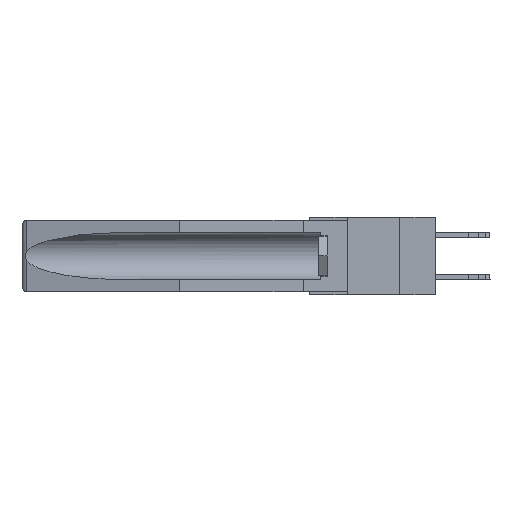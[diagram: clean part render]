
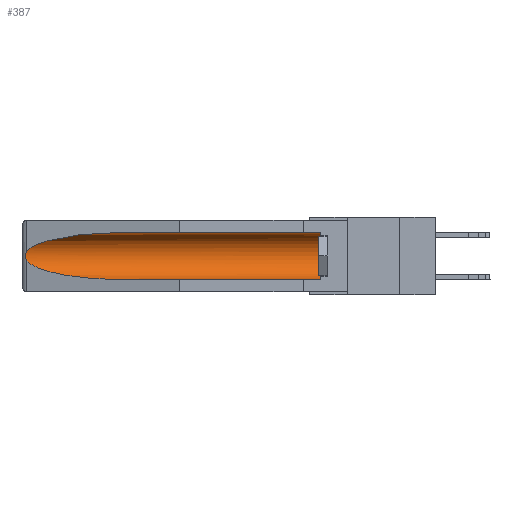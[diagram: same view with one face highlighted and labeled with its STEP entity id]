
A CAD part, left-side view. The second image highlights one B-rep face of the part: STEP entity #387.
In plain terms, the highlighted cylindrical face has radius 2.857 mm (diameter 5.715 mm), a partial arc.
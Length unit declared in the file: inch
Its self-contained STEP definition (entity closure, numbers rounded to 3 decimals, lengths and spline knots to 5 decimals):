
#278 = CARTESIAN_POINT ( 'NONE',  ( 0.155, -0.30754, -0.284 ) ) ;
#387 = ADVANCED_FACE ( 'NONE', ( #7791 ), #4352, .F. ) ;
#392 = DIRECTION ( 'NONE',  ( 0., 1., 0. ) ) ;
#547 = ORIENTED_EDGE ( 'NONE', *, *, #2767, .T. ) ;
#944 = VERTEX_POINT ( 'NONE', #14976 ) ;
#1059 = VERTEX_POINT ( 'NONE', #2539 ) ;
#2043 = CARTESIAN_POINT ( 'NONE',  ( 0.26597, 1.52961, -0.15275 ) ) ;
#2257 = VECTOR ( 'NONE', #392, 39.37008 ) ;
#2539 = CARTESIAN_POINT ( 'NONE',  ( 0.26537, 1.52718, -0.19328 ) ) ;
#2569 = EDGE_CURVE ( 'NONE', #944, #1059, #17378, .T. ) ;
#2767 = EDGE_CURVE ( 'NONE', #16362, #15933, #8404, .T. ) ;
#2847 = ORIENTED_EDGE ( 'NONE', *, *, #15312, .T. ) ;
#2925 = ORIENTED_EDGE ( 'NONE', *, *, #7594, .F. ) ;
#3388 = CARTESIAN_POINT ( 'NONE',  ( 0.2673, 1.5327, -0.16383 ) ) ;
#3452 = CARTESIAN_POINT ( 'NONE',  ( 0.2675, 1.53308, -0.17534 ) ) ;
#3769 = CARTESIAN_POINT ( 'NONE',  ( 0.21114, 1.30732, -0.059 ) ) ;
#4297 = EDGE_LOOP ( 'NONE', ( #7400, #14884, #2847, #2925, #547, #15080 ) ) ;
#4300 = EDGE_CURVE ( 'NONE', #12105, #944, #15067, .T. ) ;
#4352 = CYLINDRICAL_SURFACE ( 'NONE', #15417, 0.1125 ) ;
#4478 = DIRECTION ( 'NONE',  ( 0., 1., 0. ) ) ;
#5086 = CARTESIAN_POINT ( 'NONE',  ( 0.155, 1.07973, -0.059 ) ) ;
#5438 = CARTESIAN_POINT ( 'NONE',  ( 0.26537, 1.52718, -0.19328 ) ) ;
#7260 = DIRECTION ( 'NONE',  ( 0., 0., 1. ) ) ;
#7400 = ORIENTED_EDGE ( 'NONE', *, *, #4300, .T. ) ;
#7594 = EDGE_CURVE ( 'NONE', #16362, #12061, #15468, .T. ) ;
#7743 = CARTESIAN_POINT ( 'NONE',  ( 0.25451, 1.48313, -0.09465 ) ) ;
#7791 = FACE_OUTER_BOUND ( 'NONE', #4297, .T. ) ;
#8350 = CARTESIAN_POINT ( 'NONE',  ( 0.25451, 1.48313, -0.24835 ) ) ;
#8404 = CIRCLE ( 'NONE', #9414, 0.1125 ) ;
#9414 = AXIS2_PLACEMENT_3D ( 'NONE', #10332, #17138, #13149 ) ;
#9987 = CARTESIAN_POINT ( 'NONE',  ( 0.155, -0.30754, -0.059 ) ) ;
#10272 = CARTESIAN_POINT ( 'NONE',  ( 0.26537, 1.52718, -0.14972 ) ) ;
#10332 = CARTESIAN_POINT ( 'NONE',  ( 0.155, 0.126, -0.1715 ) ) ;
#11427 = CARTESIAN_POINT ( 'NONE',  ( 0.26537, 1.52718, -0.19328 ) ) ;
#12061 = VERTEX_POINT ( 'NONE', #16792 ) ;
#12105 = VERTEX_POINT ( 'NONE', #5086 ) ;
#12358 = CARTESIAN_POINT ( 'NONE',  ( 0.21114, 1.30732, -0.284 ) ) ;
#12684 = CARTESIAN_POINT ( 'NONE',  ( 0.155, -0.30754, -0.1715 ) ) ;
#12756 = CARTESIAN_POINT ( 'NONE',  ( 0.26655, 1.53094, -0.18657 ) ) ;
#12764 = LINE ( 'NONE', #9987, #15703 ) ;
#13149 = DIRECTION ( 'NONE',  ( 0., 0., 1. ) ) ;
#13809 = CARTESIAN_POINT ( 'NONE',  ( 0.155, 1.07973, -0.284 ) ) ;
#14308 = CARTESIAN_POINT ( 'NONE',  ( 0.2675, 1.53308, -0.16763 ) ) ;
#14505 = CARTESIAN_POINT ( 'NONE',  ( 0.155, 1.07973, -0.059 ) ) ;
#14884 = ORIENTED_EDGE ( 'NONE', *, *, #2569, .T. ) ;
#14976 = CARTESIAN_POINT ( 'NONE',  ( 0.26537, 1.52718, -0.14972 ) ) ;
#15067 =( BOUNDED_CURVE ( )  B_SPLINE_CURVE ( 3, ( #14505, #3769, #7743, #17256 ),
 .UNSPECIFIED., .F., .F. ) 
 B_SPLINE_CURVE_WITH_KNOTS ( ( 4, 4 ),
 ( 4.71239, 6.08839 ),
 .UNSPECIFIED. ) 
 CURVE ( )  GEOMETRIC_REPRESENTATION_ITEM ( )  RATIONAL_B_SPLINE_CURVE ( ( 1., 0.848, 0.848, 1. ) ) 
 REPRESENTATION_ITEM ( '' )  );
#15080 = ORIENTED_EDGE ( 'NONE', *, *, #17564, .T. ) ;
#15312 = EDGE_CURVE ( 'NONE', #1059, #12061, #16622, .T. ) ;
#15403 = CARTESIAN_POINT ( 'NONE',  ( 0.26597, 1.5296, -0.19026 ) ) ;
#15417 = AXIS2_PLACEMENT_3D ( 'NONE', #12684, #4478, #7260 ) ;
#15468 = LINE ( 'NONE', #278, #2257 ) ;
#15663 = CARTESIAN_POINT ( 'NONE',  ( 0.2673, 1.53269, -0.17917 ) ) ;
#15703 = VECTOR ( 'NONE', #16709, 39.37008 ) ;
#15933 = VERTEX_POINT ( 'NONE', #16894 ) ;
#16184 = CARTESIAN_POINT ( 'NONE',  ( 0.155, 0.126, -0.284 ) ) ;
#16362 = VERTEX_POINT ( 'NONE', #16184 ) ;
#16622 =( BOUNDED_CURVE ( )  B_SPLINE_CURVE ( 3, ( #5438, #8350, #12358, #13809 ),
 .UNSPECIFIED., .F., .F. ) 
 B_SPLINE_CURVE_WITH_KNOTS ( ( 4, 4 ),
 ( 0.1948, 1.5708 ),
 .UNSPECIFIED. ) 
 CURVE ( )  GEOMETRIC_REPRESENTATION_ITEM ( )  RATIONAL_B_SPLINE_CURVE ( ( 1., 0.848, 0.848, 1. ) ) 
 REPRESENTATION_ITEM ( '' )  );
#16709 = DIRECTION ( 'NONE',  ( 0., 1., 0. ) ) ;
#16792 = CARTESIAN_POINT ( 'NONE',  ( 0.155, 1.07973, -0.284 ) ) ;
#16894 = CARTESIAN_POINT ( 'NONE',  ( 0.155, 0.126, -0.059 ) ) ;
#17064 = CARTESIAN_POINT ( 'NONE',  ( 0.26654, 1.53092, -0.15636 ) ) ;
#17138 = DIRECTION ( 'NONE',  ( 0., -1., 0. ) ) ;
#17256 = CARTESIAN_POINT ( 'NONE',  ( 0.26537, 1.52718, -0.14972 ) ) ;
#17378 = B_SPLINE_CURVE_WITH_KNOTS ( 'NONE', 3,
 ( #10272, #2043, #17064, #3388, #14308, #3452, #15663, #12756, #15403, #11427 ),
 .UNSPECIFIED., .F., .F.,
 ( 4, 2, 2, 2, 4 ),
 ( 0., 0.00029, 0.00058, 0.00087, 0.00117 ),
 .UNSPECIFIED. ) ;
#17564 = EDGE_CURVE ( 'NONE', #15933, #12105, #12764, .T. ) ;
